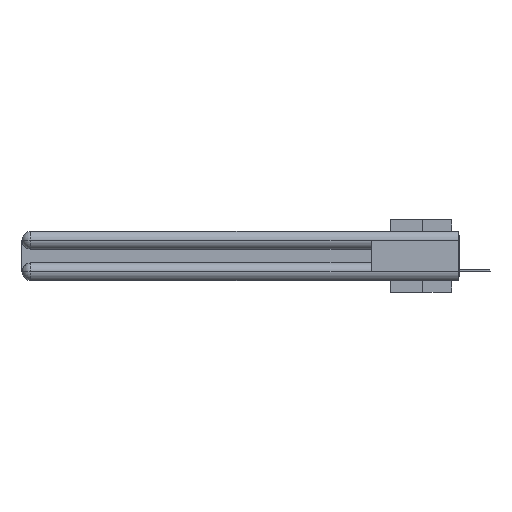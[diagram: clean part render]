
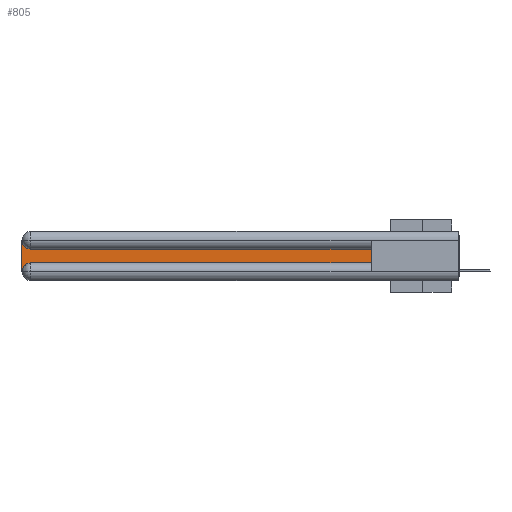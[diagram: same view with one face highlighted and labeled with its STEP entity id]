
A CAD part, left-side view. The second image highlights one B-rep face of the part: STEP entity #805.
In plain terms, the highlighted planar face has unit normal (-1, 0, 0).
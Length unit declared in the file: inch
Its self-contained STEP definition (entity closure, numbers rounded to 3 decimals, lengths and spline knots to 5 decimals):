
#90 = VECTOR ( 'NONE', #6903, 39.37008 ) ;
#805 = ADVANCED_FACE ( 'NONE', ( #21938 ), #26942, .F. ) ;
#1037 = DIRECTION ( 'NONE',  ( 1., 0., 0. ) ) ;
#1579 = CARTESIAN_POINT ( 'NONE',  ( 0.075, 0.6, -0.2175 ) ) ;
#2396 = VECTOR ( 'NONE', #12175, 39.37008 ) ;
#4350 = EDGE_CURVE ( 'NONE', #7266, #26210, #23410, .T. ) ;
#4824 = DIRECTION ( 'NONE',  ( 0., 0., -1. ) ) ;
#6567 = CARTESIAN_POINT ( 'NONE',  ( 0.075, 2.94, -0.0625 ) ) ;
#6747 = CARTESIAN_POINT ( 'NONE',  ( 0.075, 2.94, -0.2775 ) ) ;
#6903 = DIRECTION ( 'NONE',  ( 0., 1., 0. ) ) ;
#6911 = CIRCLE ( 'NONE', #18881, 0.06 ) ;
#7266 = VERTEX_POINT ( 'NONE', #1579 ) ;
#9938 = ORIENTED_EDGE ( 'NONE', *, *, #12578, .T. ) ;
#11550 = CARTESIAN_POINT ( 'NONE',  ( 0.075, 3., -0.2175 ) ) ;
#11868 = DIRECTION ( 'NONE',  ( 0., 0., -1. ) ) ;
#11906 = DIRECTION ( 'NONE',  ( 1., 0., 0. ) ) ;
#12130 = ORIENTED_EDGE ( 'NONE', *, *, #4350, .T. ) ;
#12175 = DIRECTION ( 'NONE',  ( 0., 0., 1. ) ) ;
#12568 = ORIENTED_EDGE ( 'NONE', *, *, #16356, .T. ) ;
#12578 = EDGE_CURVE ( 'NONE', #23206, #7266, #19183, .T. ) ;
#12692 = VECTOR ( 'NONE', #14419, 39.37008 ) ;
#12694 = EDGE_LOOP ( 'NONE', ( #13128, #24673, #12568, #18128, #9938, #12130 ) ) ;
#13128 = ORIENTED_EDGE ( 'NONE', *, *, #14130, .T. ) ;
#14107 = LINE ( 'NONE', #22687, #90 ) ;
#14130 = EDGE_CURVE ( 'NONE', #26210, #30013, #14107, .T. ) ;
#14419 = DIRECTION ( 'NONE',  ( 0., 0., -1. ) ) ;
#15157 = DIRECTION ( 'NONE',  ( 1., 0., 0. ) ) ;
#15190 = CARTESIAN_POINT ( 'NONE',  ( 0.075, 2.94, -0.1225 ) ) ;
#15921 = CARTESIAN_POINT ( 'NONE',  ( 0.075, 3., -0.0625 ) ) ;
#16356 = EDGE_CURVE ( 'NONE', #33739, #18958, #20140, .T. ) ;
#17608 = DIRECTION ( 'NONE',  ( 0., -1., 0. ) ) ;
#18128 = ORIENTED_EDGE ( 'NONE', *, *, #31037, .T. ) ;
#18345 = AXIS2_PLACEMENT_3D ( 'NONE', #23480, #15157, #4824 ) ;
#18533 = CIRCLE ( 'NONE', #29441, 0.06 ) ;
#18881 = AXIS2_PLACEMENT_3D ( 'NONE', #6567, #1037, #11868 ) ;
#18958 = VERTEX_POINT ( 'NONE', #31684 ) ;
#19183 = LINE ( 'NONE', #33323, #26613 ) ;
#20140 = LINE ( 'NONE', #11550, #12692 ) ;
#21938 = FACE_OUTER_BOUND ( 'NONE', #12694, .T. ) ;
#22687 = CARTESIAN_POINT ( 'NONE',  ( 0.075, 0.6, -0.1225 ) ) ;
#23206 = VERTEX_POINT ( 'NONE', #27895 ) ;
#23410 = LINE ( 'NONE', #28338, #2396 ) ;
#23480 = CARTESIAN_POINT ( 'NONE',  ( 0.075, 3., -0.1225 ) ) ;
#24673 = ORIENTED_EDGE ( 'NONE', *, *, #24897, .T. ) ;
#24897 = EDGE_CURVE ( 'NONE', #30013, #33739, #6911, .T. ) ;
#25094 = DIRECTION ( 'NONE',  ( 0., 0., -1. ) ) ;
#26210 = VERTEX_POINT ( 'NONE', #27289 ) ;
#26613 = VECTOR ( 'NONE', #17608, 39.37008 ) ;
#26942 = PLANE ( 'NONE',  #18345 ) ;
#27289 = CARTESIAN_POINT ( 'NONE',  ( 0.075, 0.6, -0.1225 ) ) ;
#27895 = CARTESIAN_POINT ( 'NONE',  ( 0.075, 2.94, -0.2175 ) ) ;
#28338 = CARTESIAN_POINT ( 'NONE',  ( 0.075, 0.6, -0.2175 ) ) ;
#29441 = AXIS2_PLACEMENT_3D ( 'NONE', #6747, #11906, #25094 ) ;
#30013 = VERTEX_POINT ( 'NONE', #15190 ) ;
#31037 = EDGE_CURVE ( 'NONE', #18958, #23206, #18533, .T. ) ;
#31684 = CARTESIAN_POINT ( 'NONE',  ( 0.075, 3., -0.2775 ) ) ;
#33323 = CARTESIAN_POINT ( 'NONE',  ( 0.075, 0.6, -0.2175 ) ) ;
#33739 = VERTEX_POINT ( 'NONE', #15921 ) ;
